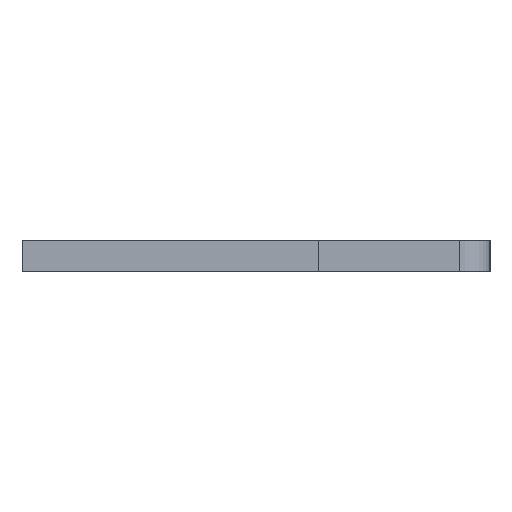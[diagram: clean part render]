
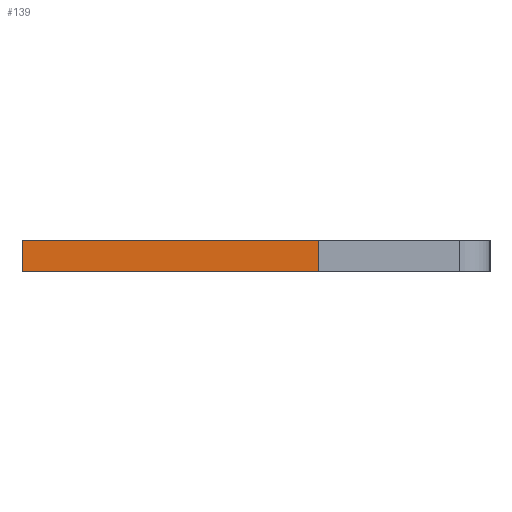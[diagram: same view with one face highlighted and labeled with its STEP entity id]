
A CAD part, left-side view. The second image highlights one B-rep face of the part: STEP entity #139.
In plain terms, the highlighted face is planar.
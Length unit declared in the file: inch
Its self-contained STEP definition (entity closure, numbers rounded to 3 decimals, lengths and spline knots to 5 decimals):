
#51 = VECTOR ( 'NONE', #60, 39.37008 ) ;
#54 = VECTOR ( 'NONE', #1318, 39.37008 ) ;
#57 = PLANE ( 'NONE',  #616 ) ;
#60 = DIRECTION ( 'NONE',  ( 0., 1., 0. ) ) ;
#76 = EDGE_CURVE ( 'NONE', #684, #1193, #397, .T. ) ;
#94 = ORIENTED_EDGE ( 'NONE', *, *, #1211, .F. ) ;
#137 = VECTOR ( 'NONE', #365, 39.37008 ) ;
#139 = ADVANCED_FACE ( 'NONE', ( #882 ), #57, .F. ) ;
#238 = CARTESIAN_POINT ( 'NONE',  ( 0.01, -0.04, -0.04 ) ) ;
#275 = EDGE_CURVE ( 'NONE', #1193, #1037, #373, .T. ) ;
#338 = LINE ( 'NONE', #663, #54 ) ;
#365 = DIRECTION ( 'NONE',  ( -1., 0., 0. ) ) ;
#373 = LINE ( 'NONE', #379, #51 ) ;
#377 = CARTESIAN_POINT ( 'NONE',  ( -0.01, 0.15, -0.04 ) ) ;
#379 = CARTESIAN_POINT ( 'NONE',  ( -0.01, 0.15, -0.04 ) ) ;
#397 = LINE ( 'NONE', #572, #600 ) ;
#475 = CARTESIAN_POINT ( 'NONE',  ( 0.01, 0.15, -0.04 ) ) ;
#496 = CARTESIAN_POINT ( 'NONE',  ( 0.01, 0.15, -0.04 ) ) ;
#572 = CARTESIAN_POINT ( 'NONE',  ( 0.01, -0.04, -0.04 ) ) ;
#600 = VECTOR ( 'NONE', #1117, 39.37008 ) ;
#616 = AXIS2_PLACEMENT_3D ( 'NONE', #496, #1029, #814 ) ;
#663 = CARTESIAN_POINT ( 'NONE',  ( 0.01, 0.15, -0.04 ) ) ;
#675 = CARTESIAN_POINT ( 'NONE',  ( -0.01, -0.04, -0.04 ) ) ;
#684 = VERTEX_POINT ( 'NONE', #238 ) ;
#711 = LINE ( 'NONE', #475, #137 ) ;
#723 = EDGE_CURVE ( 'NONE', #867, #1037, #711, .T. ) ;
#797 = EDGE_LOOP ( 'NONE', ( #978, #1282, #94, #855 ) ) ;
#814 = DIRECTION ( 'NONE',  ( 1., 0., 0. ) ) ;
#855 = ORIENTED_EDGE ( 'NONE', *, *, #76, .T. ) ;
#867 = VERTEX_POINT ( 'NONE', #1322 ) ;
#882 = FACE_OUTER_BOUND ( 'NONE', #797, .T. ) ;
#978 = ORIENTED_EDGE ( 'NONE', *, *, #275, .T. ) ;
#1029 = DIRECTION ( 'NONE',  ( 0., 0., 1. ) ) ;
#1037 = VERTEX_POINT ( 'NONE', #377 ) ;
#1117 = DIRECTION ( 'NONE',  ( -1., 0., 0. ) ) ;
#1193 = VERTEX_POINT ( 'NONE', #675 ) ;
#1211 = EDGE_CURVE ( 'NONE', #684, #867, #338, .T. ) ;
#1282 = ORIENTED_EDGE ( 'NONE', *, *, #723, .F. ) ;
#1318 = DIRECTION ( 'NONE',  ( 0., 1., 0. ) ) ;
#1322 = CARTESIAN_POINT ( 'NONE',  ( 0.01, 0.15, -0.04 ) ) ;
